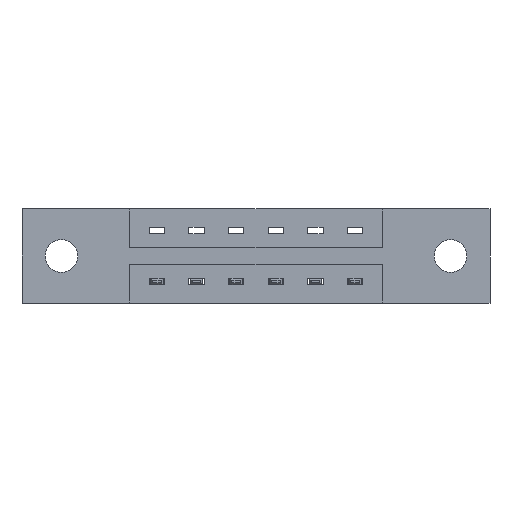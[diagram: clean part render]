
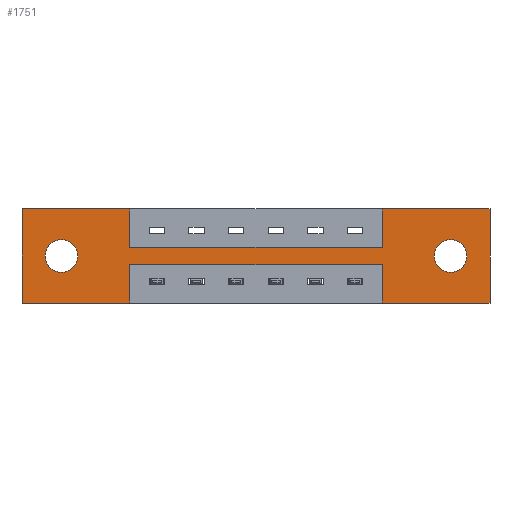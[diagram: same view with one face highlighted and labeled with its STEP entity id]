
A CAD part, front view. The second image highlights one B-rep face of the part: STEP entity #1751.
In plain terms, the highlighted planar face has unit normal (0, -1, 0).
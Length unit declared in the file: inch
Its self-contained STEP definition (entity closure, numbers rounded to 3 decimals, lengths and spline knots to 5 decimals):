
#308 = FACE_OUTER_BOUND ( 'NONE', #7963, .T. ) ;
#344 = AXIS2_PLACEMENT_3D ( 'NONE', #1157, #7511, #7500 ) ;
#422 = LINE ( 'NONE', #4655, #722 ) ;
#434 = VERTEX_POINT ( 'NONE', #4275 ) ;
#485 = DIRECTION ( 'NONE',  ( 0., 0., -1. ) ) ;
#645 = CARTESIAN_POINT ( 'NONE',  ( 0., 0., 0. ) ) ;
#663 = VERTEX_POINT ( 'NONE', #5560 ) ;
#673 = VERTEX_POINT ( 'NONE', #5858 ) ;
#692 = DIRECTION ( 'NONE',  ( 1., 0., 0. ) ) ;
#703 = DIRECTION ( 'NONE',  ( 0., 0., 1. ) ) ;
#722 = VECTOR ( 'NONE', #692, 39.37008 ) ;
#748 = ORIENTED_EDGE ( 'NONE', *, *, #6090, .T. ) ;
#875 = CARTESIAN_POINT ( 'NONE',  ( 0.425, 0., -0.22 ) ) ;
#888 = DIRECTION ( 'NONE',  ( 0., 0., -1. ) ) ;
#1097 = EDGE_LOOP ( 'NONE', ( #2269, #2396 ) ) ;
#1157 = CARTESIAN_POINT ( 'NONE',  ( 0.155, 0., -0.185 ) ) ;
#1185 = DIRECTION ( 'NONE',  ( -1., 0., 0. ) ) ;
#1460 = VECTOR ( 'NONE', #3413, 39.37008 ) ;
#1645 = CARTESIAN_POINT ( 'NONE',  ( 1.417, 0., -0.37 ) ) ;
#1731 = VECTOR ( 'NONE', #485, 39.37008 ) ;
#1751 = ADVANCED_FACE ( 'NONE', ( #5905, #2505, #308 ), #5831, .T. ) ;
#1792 = ORIENTED_EDGE ( 'NONE', *, *, #2660, .F. ) ;
#1827 = DIRECTION ( 'NONE',  ( -1., 0., 0. ) ) ;
#2002 = DIRECTION ( 'NONE',  ( 0., 1., 0. ) ) ;
#2078 = CARTESIAN_POINT ( 'NONE',  ( 1.417, 0., 0. ) ) ;
#2171 = EDGE_CURVE ( 'NONE', #7329, #3928, #4864, .T. ) ;
#2226 = EDGE_CURVE ( 'NONE', #6432, #434, #7692, .T. ) ;
#2231 = EDGE_CURVE ( 'NONE', #663, #4622, #422, .T. ) ;
#2236 = CARTESIAN_POINT ( 'NONE',  ( 1.687, 0., -0.185 ) ) ;
#2268 = DIRECTION ( 'NONE',  ( 0., 0., 1. ) ) ;
#2269 = ORIENTED_EDGE ( 'NONE', *, *, #6650, .T. ) ;
#2285 = ORIENTED_EDGE ( 'NONE', *, *, #5099, .F. ) ;
#2327 = ORIENTED_EDGE ( 'NONE', *, *, #2231, .F. ) ;
#2358 = EDGE_LOOP ( 'NONE', ( #2804, #748 ) ) ;
#2369 = ORIENTED_EDGE ( 'NONE', *, *, #2226, .F. ) ;
#2372 = DIRECTION ( 'NONE',  ( 0., 0., -1. ) ) ;
#2396 = ORIENTED_EDGE ( 'NONE', *, *, #3026, .T. ) ;
#2505 = FACE_BOUND ( 'NONE', #2358, .T. ) ;
#2544 = VECTOR ( 'NONE', #8056, 39.37008 ) ;
#2548 = DIRECTION ( 'NONE',  ( 0., 0., -1. ) ) ;
#2576 = VECTOR ( 'NONE', #2268, 39.37008 ) ;
#2590 = VECTOR ( 'NONE', #1827, 39.37008 ) ;
#2625 = CARTESIAN_POINT ( 'NONE',  ( 1.417, 0., -0.37 ) ) ;
#2627 = CARTESIAN_POINT ( 'NONE',  ( 1.687, 0., -0.185 ) ) ;
#2630 = ORIENTED_EDGE ( 'NONE', *, *, #7313, .F. ) ;
#2660 = EDGE_CURVE ( 'NONE', #434, #7329, #4444, .T. ) ;
#2670 = ORIENTED_EDGE ( 'NONE', *, *, #7476, .F. ) ;
#2711 = CARTESIAN_POINT ( 'NONE',  ( 1.842, 0., 0. ) ) ;
#2804 = ORIENTED_EDGE ( 'NONE', *, *, #4575, .T. ) ;
#2824 = LINE ( 'NONE', #8783, #2590 ) ;
#2882 = CARTESIAN_POINT ( 'NONE',  ( 0.425, 0., 0. ) ) ;
#2939 = CARTESIAN_POINT ( 'NONE',  ( 0., 0., -0.37 ) ) ;
#2971 = DIRECTION ( 'NONE',  ( 0., 0., -1. ) ) ;
#2998 = CARTESIAN_POINT ( 'NONE',  ( 0.155, 0., -0.121 ) ) ;
#3021 = CARTESIAN_POINT ( 'NONE',  ( 0.425, 0., 0. ) ) ;
#3026 = EDGE_CURVE ( 'NONE', #3438, #5172, #4849, .T. ) ;
#3189 = CARTESIAN_POINT ( 'NONE',  ( 0.155, 0., -0.249 ) ) ;
#3413 = DIRECTION ( 'NONE',  ( 0., 0., -1. ) ) ;
#3422 = CARTESIAN_POINT ( 'NONE',  ( 0., 0., 0. ) ) ;
#3426 = LINE ( 'NONE', #2711, #1460 ) ;
#3438 = VERTEX_POINT ( 'NONE', #8119 ) ;
#3478 = VERTEX_POINT ( 'NONE', #3189 ) ;
#3531 = DIRECTION ( 'NONE',  ( 1., 0., 0. ) ) ;
#3542 = EDGE_CURVE ( 'NONE', #5973, #6182, #2824, .T. ) ;
#3577 = ORIENTED_EDGE ( 'NONE', *, *, #6598, .F. ) ;
#3597 = CARTESIAN_POINT ( 'NONE',  ( 0.425, 0., -0.37 ) ) ;
#3645 = DIRECTION ( 'NONE',  ( 0., -1., 0. ) ) ;
#3732 = VECTOR ( 'NONE', #2548, 39.37008 ) ;
#3737 = ORIENTED_EDGE ( 'NONE', *, *, #4100, .F. ) ;
#3841 = DIRECTION ( 'NONE',  ( 0., 0., 1. ) ) ;
#3846 = DIRECTION ( 'NONE',  ( 0., 1., 0. ) ) ;
#3862 = CARTESIAN_POINT ( 'NONE',  ( 0.155, 0., -0.185 ) ) ;
#3928 = VERTEX_POINT ( 'NONE', #2882 ) ;
#3955 = ORIENTED_EDGE ( 'NONE', *, *, #4543, .F. ) ;
#4100 = EDGE_CURVE ( 'NONE', #8820, #6097, #5967, .T. ) ;
#4275 = CARTESIAN_POINT ( 'NONE',  ( 0., 0., -0.37 ) ) ;
#4394 = LINE ( 'NONE', #2078, #2544 ) ;
#4424 = LINE ( 'NONE', #2625, #2576 ) ;
#4444 = LINE ( 'NONE', #8585, #7682 ) ;
#4463 = EDGE_CURVE ( 'NONE', #6775, #673, #8415, .T. ) ;
#4543 = EDGE_CURVE ( 'NONE', #6097, #5973, #4424, .T. ) ;
#4575 = EDGE_CURVE ( 'NONE', #5129, #3478, #7662, .T. ) ;
#4622 = VERTEX_POINT ( 'NONE', #5407 ) ;
#4655 = CARTESIAN_POINT ( 'NONE',  ( 0.425, 0., -0.15 ) ) ;
#4697 = CARTESIAN_POINT ( 'NONE',  ( 1.842, 0., -0.37 ) ) ;
#4830 = CIRCLE ( 'NONE', #344, 0.064 ) ;
#4849 = CIRCLE ( 'NONE', #5231, 0.064 ) ;
#4864 = LINE ( 'NONE', #645, #8061 ) ;
#5099 = EDGE_CURVE ( 'NONE', #3928, #663, #8860, .T. ) ;
#5129 = VERTEX_POINT ( 'NONE', #2998 ) ;
#5172 = VERTEX_POINT ( 'NONE', #8886 ) ;
#5225 = CIRCLE ( 'NONE', #7470, 0.064 ) ;
#5231 = AXIS2_PLACEMENT_3D ( 'NONE', #2627, #2002, #888 ) ;
#5407 = CARTESIAN_POINT ( 'NONE',  ( 1.417, 0., -0.15 ) ) ;
#5509 = CARTESIAN_POINT ( 'NONE',  ( 0.425, 0., -0.37 ) ) ;
#5560 = CARTESIAN_POINT ( 'NONE',  ( 0.425, 0., -0.15 ) ) ;
#5569 = DIRECTION ( 'NONE',  ( 1., 0., 0. ) ) ;
#5729 = CARTESIAN_POINT ( 'NONE',  ( 1.417, 0., 0. ) ) ;
#5753 = VECTOR ( 'NONE', #1185, 39.37008 ) ;
#5824 = DIRECTION ( 'NONE',  ( -1., 0., 0. ) ) ;
#5831 = PLANE ( 'NONE',  #7200 ) ;
#5858 = CARTESIAN_POINT ( 'NONE',  ( 1.842, 0., 0. ) ) ;
#5905 = FACE_BOUND ( 'NONE', #1097, .T. ) ;
#5967 = LINE ( 'NONE', #7995, #5753 ) ;
#5973 = VERTEX_POINT ( 'NONE', #7215 ) ;
#5986 = VECTOR ( 'NONE', #5824, 39.37008 ) ;
#6090 = EDGE_CURVE ( 'NONE', #3478, #5129, #4830, .T. ) ;
#6097 = VERTEX_POINT ( 'NONE', #1645 ) ;
#6182 = VERTEX_POINT ( 'NONE', #875 ) ;
#6283 = ORIENTED_EDGE ( 'NONE', *, *, #4463, .F. ) ;
#6432 = VERTEX_POINT ( 'NONE', #5509 ) ;
#6598 = EDGE_CURVE ( 'NONE', #6182, #6432, #6962, .T. ) ;
#6650 = EDGE_CURVE ( 'NONE', #5172, #3438, #5225, .T. ) ;
#6699 = ORIENTED_EDGE ( 'NONE', *, *, #3542, .F. ) ;
#6773 = VECTOR ( 'NONE', #5569, 39.37008 ) ;
#6775 = VERTEX_POINT ( 'NONE', #5729 ) ;
#6959 = DIRECTION ( 'NONE',  ( 0., 1., 0. ) ) ;
#6962 = LINE ( 'NONE', #3597, #1731 ) ;
#7200 = AXIS2_PLACEMENT_3D ( 'NONE', #2939, #3645, #2372 ) ;
#7215 = CARTESIAN_POINT ( 'NONE',  ( 1.417, 0., -0.22 ) ) ;
#7269 = ORIENTED_EDGE ( 'NONE', *, *, #2171, .F. ) ;
#7313 = EDGE_CURVE ( 'NONE', #673, #8820, #3426, .T. ) ;
#7329 = VERTEX_POINT ( 'NONE', #8589 ) ;
#7367 = AXIS2_PLACEMENT_3D ( 'NONE', #3862, #3846, #3841 ) ;
#7470 = AXIS2_PLACEMENT_3D ( 'NONE', #2236, #6959, #2971 ) ;
#7476 = EDGE_CURVE ( 'NONE', #4622, #6775, #4394, .T. ) ;
#7500 = DIRECTION ( 'NONE',  ( 0., 0., 1. ) ) ;
#7511 = DIRECTION ( 'NONE',  ( 0., 1., 0. ) ) ;
#7662 = CIRCLE ( 'NONE', #7367, 0.064 ) ;
#7682 = VECTOR ( 'NONE', #703, 39.37008 ) ;
#7692 = LINE ( 'NONE', #8382, #5986 ) ;
#7963 = EDGE_LOOP ( 'NONE', ( #3577, #6699, #3955, #3737, #2630, #6283, #2670, #2327, #2285, #7269, #1792, #2369 ) ) ;
#7995 = CARTESIAN_POINT ( 'NONE',  ( 0., 0., -0.37 ) ) ;
#8056 = DIRECTION ( 'NONE',  ( 0., 0., 1. ) ) ;
#8061 = VECTOR ( 'NONE', #3531, 39.37008 ) ;
#8119 = CARTESIAN_POINT ( 'NONE',  ( 1.687, 0., -0.249 ) ) ;
#8382 = CARTESIAN_POINT ( 'NONE',  ( 0., 0., -0.37 ) ) ;
#8415 = LINE ( 'NONE', #3422, #6773 ) ;
#8585 = CARTESIAN_POINT ( 'NONE',  ( 0., 0., 0. ) ) ;
#8589 = CARTESIAN_POINT ( 'NONE',  ( 0., 0., 0. ) ) ;
#8783 = CARTESIAN_POINT ( 'NONE',  ( 0.425, 0., -0.22 ) ) ;
#8820 = VERTEX_POINT ( 'NONE', #4697 ) ;
#8860 = LINE ( 'NONE', #3021, #3732 ) ;
#8886 = CARTESIAN_POINT ( 'NONE',  ( 1.687, 0., -0.121 ) ) ;
